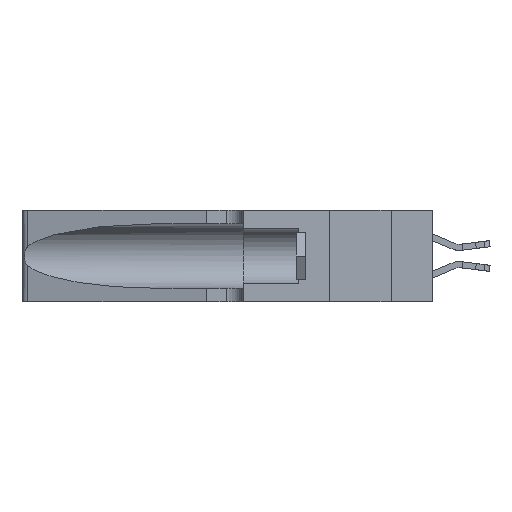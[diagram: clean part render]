
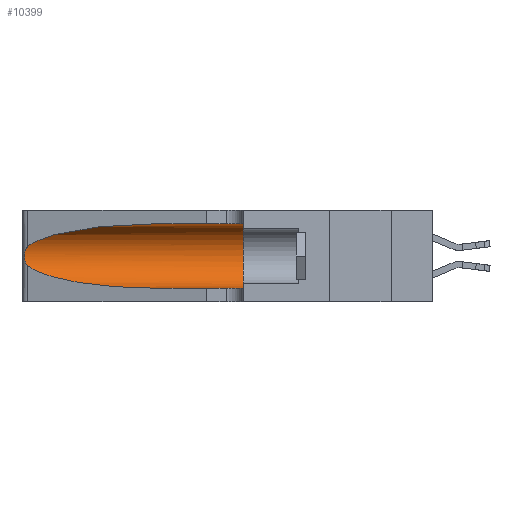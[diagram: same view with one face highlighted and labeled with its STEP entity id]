
A CAD part, left-side view. The second image highlights one B-rep face of the part: STEP entity #10399.
In plain terms, the highlighted cylindrical face has radius 3.308 mm (diameter 6.617 mm), a partial arc.
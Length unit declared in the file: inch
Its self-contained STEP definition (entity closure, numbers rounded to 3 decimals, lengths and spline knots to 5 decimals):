
#10 =( BOUNDED_CURVE ( )  B_SPLINE_CURVE ( 3, ( #27916, #14781, #23306, #3830 ),
 .UNSPECIFIED., .F., .F. ) 
 B_SPLINE_CURVE_WITH_KNOTS ( ( 4, 4 ),
 ( 1.5708, 2.84003 ),
 .UNSPECIFIED. ) 
 CURVE ( )  GEOMETRIC_REPRESENTATION_ITEM ( )  RATIONAL_B_SPLINE_CURVE ( ( 1., 0.87, 0.87, 1. ) ) 
 REPRESENTATION_ITEM ( '' )  );
#128 = CARTESIAN_POINT ( 'NONE',  ( 0.18966, 0.96281, 0.05475 ) ) ;
#561 = CARTESIAN_POINT ( 'NONE',  ( 0.25856, 1.23593, 0.16098 ) ) ;
#743 = CARTESIAN_POINT ( 'NONE',  ( 0.25555, 1.22993, 0.14849 ) ) ;
#754 = CARTESIAN_POINT ( 'NONE',  ( 0.1305, 1.61858, 0.05475 ) ) ;
#934 = CARTESIAN_POINT ( 'NONE',  ( 0.25487, 1.22718, 0.14631 ) ) ;
#1534 = EDGE_CURVE ( 'NONE', #26590, #3099, #8898, .T. ) ;
#2050 = CARTESIAN_POINT ( 'NONE',  ( 0.1305, 0.72297, 0.05475 ) ) ;
#3099 = VERTEX_POINT ( 'NONE', #18274 ) ;
#3830 = CARTESIAN_POINT ( 'NONE',  ( 0.25487, 1.22718, 0.22369 ) ) ;
#5065 = CARTESIAN_POINT ( 'NONE',  ( 0.25639, 1.23186, 0.15144 ) ) ;
#5167 = CARTESIAN_POINT ( 'NONE',  ( 0.25854, 1.2359, 0.20912 ) ) ;
#5273 = VERTEX_POINT ( 'NONE', #23736 ) ;
#5320 = DIRECTION ( 'NONE',  ( 0., -1., 0. ) ) ;
#5479 = CARTESIAN_POINT ( 'NONE',  ( 0.25487, 1.22718, 0.22369 ) ) ;
#6632 = ORIENTED_EDGE ( 'NONE', *, *, #12795, .T. ) ;
#6646 = CARTESIAN_POINT ( 'NONE',  ( 0.25487, 1.22718, 0.14631 ) ) ;
#6967 = LINE ( 'NONE', #754, #18662 ) ;
#8067 = VECTOR ( 'NONE', #26977, 39.37008 ) ;
#8898 = CIRCLE ( 'NONE', #18931, 0.13025 ) ;
#9080 = VERTEX_POINT ( 'NONE', #5479 ) ;
#9360 =( BOUNDED_CURVE ( )  B_SPLINE_CURVE ( 3, ( #19721, #11084, #128, #2050 ),
 .UNSPECIFIED., .F., .T. ) 
 B_SPLINE_CURVE_WITH_KNOTS ( ( 4, 4 ),
 ( 3.44316, 4.71239 ),
 .UNSPECIFIED. ) 
 CURVE ( )  GEOMETRIC_REPRESENTATION_ITEM ( )  RATIONAL_B_SPLINE_CURVE ( ( 1., 0.87, 0.87, 1. ) ) 
 REPRESENTATION_ITEM ( '' )  );
#9624 = EDGE_CURVE ( 'NONE', #23422, #3099, #6967, .T. ) ;
#9702 = CARTESIAN_POINT ( 'NONE',  ( 0.1305, 1.61858, 0.31525 ) ) ;
#9871 = B_SPLINE_CURVE_WITH_KNOTS ( 'NONE', 3,
 ( #26865, #11898, #22833, #26961, #5167, #13735, #14114, #18237, #27055, #561, #13918, #5065, #743, #934 ),
 .UNSPECIFIED., .F., .F.,
 ( 4, 2, 2, 2, 2, 2, 4 ),
 ( 0., 0.00027, 0.00053, 0.00107, 0.0016, 0.00187, 0.00214 ),
 .UNSPECIFIED. ) ;
#10399 = ADVANCED_FACE ( 'NONE', ( #14158 ), #13485, .F. ) ;
#11084 = CARTESIAN_POINT ( 'NONE',  ( 0.2373, 1.15595, 0.08982 ) ) ;
#11367 = AXIS2_PLACEMENT_3D ( 'NONE', #22620, #5320, #25497 ) ;
#11813 = EDGE_CURVE ( 'NONE', #5273, #9080, #10, .T. ) ;
#11898 = CARTESIAN_POINT ( 'NONE',  ( 0.25555, 1.22994, 0.2215 ) ) ;
#12754 = VERTEX_POINT ( 'NONE', #6646 ) ;
#12795 = EDGE_CURVE ( 'NONE', #12754, #23422, #9360, .T. ) ;
#13485 = CYLINDRICAL_SURFACE ( 'NONE', #11367, 0.13025 ) ;
#13499 = EDGE_LOOP ( 'NONE', ( #20616, #27087, #6632, #14463, #19961, #17127 ) ) ;
#13735 = CARTESIAN_POINT ( 'NONE',  ( 0.26018, 1.23835, 0.19895 ) ) ;
#13918 = CARTESIAN_POINT ( 'NONE',  ( 0.25789, 1.23486, 0.15765 ) ) ;
#14114 = CARTESIAN_POINT ( 'NONE',  ( 0.26075, 1.23896, 0.19203 ) ) ;
#14158 = FACE_OUTER_BOUND ( 'NONE', #13499, .T. ) ;
#14463 = ORIENTED_EDGE ( 'NONE', *, *, #9624, .T. ) ;
#14781 = CARTESIAN_POINT ( 'NONE',  ( 0.18966, 0.96281, 0.31525 ) ) ;
#15514 = DIRECTION ( 'NONE',  ( 0., 1., 0. ) ) ;
#15790 = CARTESIAN_POINT ( 'NONE',  ( 0.1305, 0.35, 0.31525 ) ) ;
#15880 = CARTESIAN_POINT ( 'NONE',  ( 0.1305, 0.72297, 0.05475 ) ) ;
#17127 = ORIENTED_EDGE ( 'NONE', *, *, #23579, .F. ) ;
#18237 = CARTESIAN_POINT ( 'NONE',  ( 0.26075, 1.23896, 0.178 ) ) ;
#18274 = CARTESIAN_POINT ( 'NONE',  ( 0.1305, 0.35, 0.05475 ) ) ;
#18662 = VECTOR ( 'NONE', #20365, 39.37008 ) ;
#18931 = AXIS2_PLACEMENT_3D ( 'NONE', #26800, #15514, #26707 ) ;
#19721 = CARTESIAN_POINT ( 'NONE',  ( 0.25487, 1.22718, 0.14631 ) ) ;
#19961 = ORIENTED_EDGE ( 'NONE', *, *, #1534, .F. ) ;
#20365 = DIRECTION ( 'NONE',  ( 0., -1., 0. ) ) ;
#20616 = ORIENTED_EDGE ( 'NONE', *, *, #11813, .T. ) ;
#22620 = CARTESIAN_POINT ( 'NONE',  ( 0.1305, 1.61858, 0.185 ) ) ;
#22833 = CARTESIAN_POINT ( 'NONE',  ( 0.25639, 1.23184, 0.21858 ) ) ;
#23168 = LINE ( 'NONE', #9702, #8067 ) ;
#23306 = CARTESIAN_POINT ( 'NONE',  ( 0.2373, 1.15595, 0.28018 ) ) ;
#23422 = VERTEX_POINT ( 'NONE', #15880 ) ;
#23579 = EDGE_CURVE ( 'NONE', #5273, #26590, #23168, .T. ) ;
#23736 = CARTESIAN_POINT ( 'NONE',  ( 0.1305, 0.72297, 0.31525 ) ) ;
#25497 = DIRECTION ( 'NONE',  ( 0., 0., -1. ) ) ;
#26590 = VERTEX_POINT ( 'NONE', #15790 ) ;
#26707 = DIRECTION ( 'NONE',  ( 0., 0., 1. ) ) ;
#26800 = CARTESIAN_POINT ( 'NONE',  ( 0.1305, 0.35, 0.185 ) ) ;
#26865 = CARTESIAN_POINT ( 'NONE',  ( 0.25487, 1.22718, 0.22369 ) ) ;
#26961 = CARTESIAN_POINT ( 'NONE',  ( 0.25787, 1.23484, 0.2124 ) ) ;
#26977 = DIRECTION ( 'NONE',  ( 0., -1., 0. ) ) ;
#27055 = CARTESIAN_POINT ( 'NONE',  ( 0.26017, 1.23833, 0.17102 ) ) ;
#27087 = ORIENTED_EDGE ( 'NONE', *, *, #27360, .T. ) ;
#27360 = EDGE_CURVE ( 'NONE', #9080, #12754, #9871, .T. ) ;
#27916 = CARTESIAN_POINT ( 'NONE',  ( 0.1305, 0.72297, 0.31525 ) ) ;
